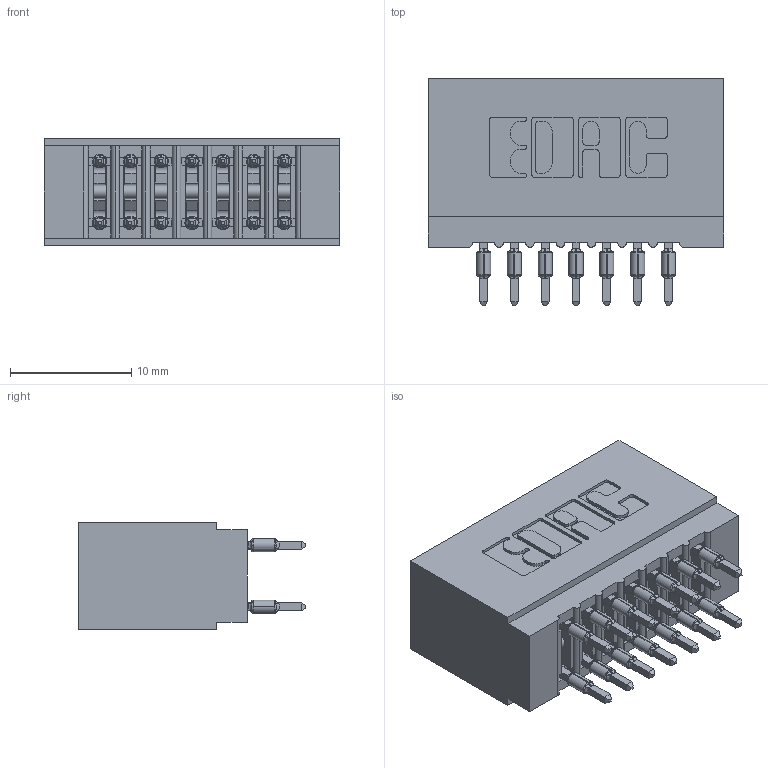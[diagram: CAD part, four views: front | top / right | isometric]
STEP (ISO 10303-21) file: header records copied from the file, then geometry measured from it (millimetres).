
FILE_DESCRIPTION (( 'STEP AP203' ), '1' );
FILE_NAME ('725-014-560-201.STEP', '2026-02-24T16:41:13', ( '' ), ( '' ), 'SwSTEP 2.0', 'SolidWorks 2023', '' );
FILE_SCHEMA (( 'CONFIG_CONTROL_DESIGN' ));
Length unit declared in the file: millimetre
Products named in the file (3): 745-292-001_560; 725 Part_Insulator Option - 01; 725-014-560-201
Assembly tree (15 placements, depth 2):
  725-014-560-201
    725 Part_Insulator Option - 01
    745-292-001_560  x14
Bounding box: 24.38 x 18.8 x 8.89 mm (x, y, z)
Volume: 2161.7 mm3; surface area: 4038 mm2
Topology: 15 solids, 15 shells, 1474 faces, 4027 edges, 2562 vertices
Faces by surface type: plane 769, cylinder 341, bspline 280, torus 84
Entity records: 16850 total; most frequent: CARTESIAN_POINT 3437, ORIENTED_EDGE 2802, DIRECTION 2485, EDGE_CURVE 1401, LINE 1169, VECTOR 1169, VERTEX_POINT 898, AXIS2_PLACEMENT_3D 658
